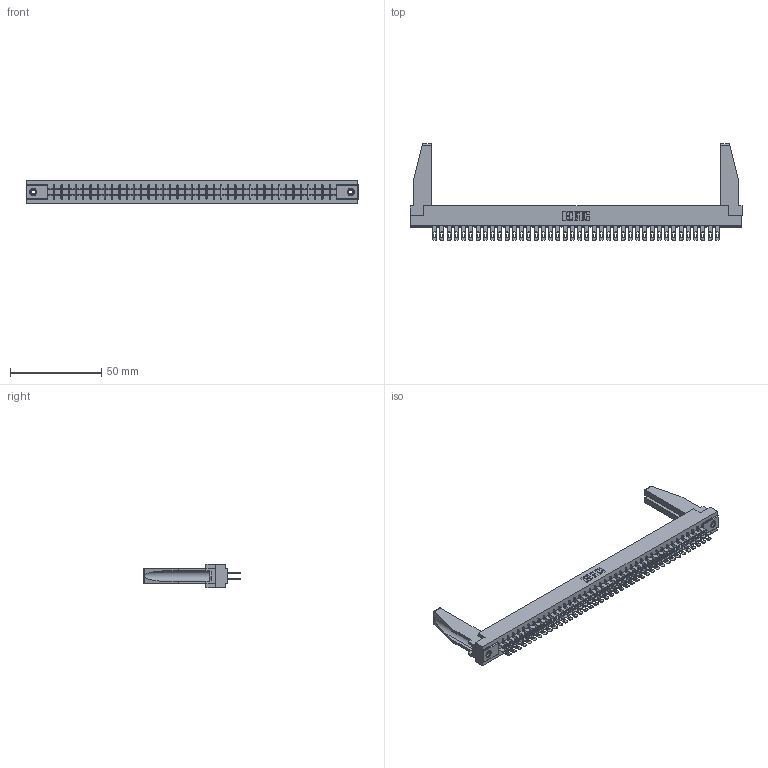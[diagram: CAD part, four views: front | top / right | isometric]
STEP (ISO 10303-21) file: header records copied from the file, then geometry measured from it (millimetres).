
FILE_DESCRIPTION (( 'STEP AP203' ), '1' );
FILE_NAME ('355-080-500-278.STEP', '2019-09-13T14:19:38', ( '' ), ( '' ), 'SwSTEP 2.0', 'SolidWorks 2016', '' );
FILE_SCHEMA (( 'CONFIG_CONTROL_DESIGN' ));
Length unit declared in the file: inch
Products named in the file (5): 305-290-001_500; 355-080-500-278; 305 Part_.156 Dia; 307-220-078; 345-250-001_345-250-001-102
Assembly tree (85 placements, depth 2):
  355-080-500-278
    305 Part_.156 Dia
    305-290-001_500  x80
    345-250-001_345-250-001-102  x2
    307-220-078  x2
Bounding box: 181.51 x 52.88 x 12.7 mm (x, y, z)
Volume: 23157.7 mm3; surface area: 29741.8 mm2
Topology: 85 solids, 85 shells, 4246 faces, 12126 edges, 7860 vertices
Faces by surface type: plane 2392, cylinder 1678, sphere 160, cone 12, torus 4
Entity records: 46014 total; most frequent: CARTESIAN_POINT 7620, ORIENTED_EDGE 7522, DIRECTION 7333, EDGE_CURVE 3761, VECTOR 3035, LINE 3035, VERTEX_POINT 2394, AXIS2_PLACEMENT_3D 2149
